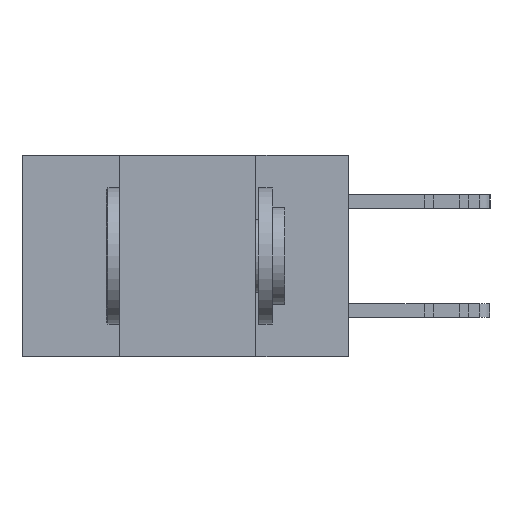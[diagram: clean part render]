
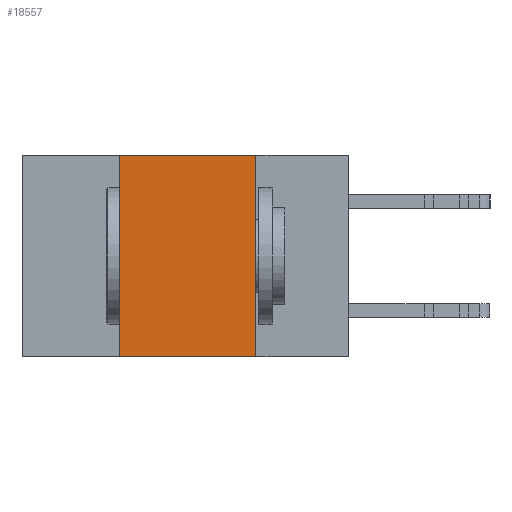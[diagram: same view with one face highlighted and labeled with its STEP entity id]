
A CAD part, left-side view. The second image highlights one B-rep face of the part: STEP entity #18557.
In plain terms, the highlighted planar face has unit normal (-1, 0, 0).
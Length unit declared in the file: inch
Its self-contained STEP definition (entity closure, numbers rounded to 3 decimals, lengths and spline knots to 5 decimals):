
#226 = LINE ( 'NONE', #10860, #3013 ) ;
#1134 = VERTEX_POINT ( 'NONE', #13275 ) ;
#3013 = VECTOR ( 'NONE', #19260, 39.37008 ) ;
#3065 = PLANE ( 'NONE',  #15069 ) ;
#3851 = EDGE_CURVE ( 'NONE', #1134, #13540, #17371, .T. ) ;
#4507 = VECTOR ( 'NONE', #18139, 39.37008 ) ;
#5438 = LINE ( 'NONE', #26823, #4507 ) ;
#6493 = ORIENTED_EDGE ( 'NONE', *, *, #16895, .F. ) ;
#6726 = ORIENTED_EDGE ( 'NONE', *, *, #10129, .F. ) ;
#6945 = DIRECTION ( 'NONE',  ( 1., 0., 0. ) ) ;
#7087 = DIRECTION ( 'NONE',  ( 0., 0., -1. ) ) ;
#8950 = VERTEX_POINT ( 'NONE', #26075 ) ;
#10129 = EDGE_CURVE ( 'NONE', #21380, #13540, #226, .T. ) ;
#10860 = CARTESIAN_POINT ( 'NONE',  ( 0., 0.17, -0.37 ) ) ;
#11260 = CARTESIAN_POINT ( 'NONE',  ( 0., 0.17, 0. ) ) ;
#11976 = ORIENTED_EDGE ( 'NONE', *, *, #14223, .F. ) ;
#12241 = ORIENTED_EDGE ( 'NONE', *, *, #3851, .T. ) ;
#12356 = VECTOR ( 'NONE', #23181, 39.37008 ) ;
#13275 = CARTESIAN_POINT ( 'NONE',  ( 0., 0.42, -0.37 ) ) ;
#13380 = CARTESIAN_POINT ( 'NONE',  ( 0., 0.6, -0.37 ) ) ;
#13540 = VERTEX_POINT ( 'NONE', #27226 ) ;
#14223 = EDGE_CURVE ( 'NONE', #8950, #21380, #21539, .T. ) ;
#15069 = AXIS2_PLACEMENT_3D ( 'NONE', #25850, #6945, #7087 ) ;
#16895 = EDGE_CURVE ( 'NONE', #1134, #8950, #5438, .T. ) ;
#17122 = CARTESIAN_POINT ( 'NONE',  ( 0., 0.6, 0. ) ) ;
#17371 = LINE ( 'NONE', #13380, #23791 ) ;
#18139 = DIRECTION ( 'NONE',  ( 0., 0., 1. ) ) ;
#18557 = ADVANCED_FACE ( 'NONE', ( #25994 ), #3065, .F. ) ;
#19260 = DIRECTION ( 'NONE',  ( 0., 0., -1. ) ) ;
#21380 = VERTEX_POINT ( 'NONE', #11260 ) ;
#21509 = DIRECTION ( 'NONE',  ( 0., -1., 0. ) ) ;
#21539 = LINE ( 'NONE', #17122, #12356 ) ;
#23181 = DIRECTION ( 'NONE',  ( 0., -1., 0. ) ) ;
#23791 = VECTOR ( 'NONE', #21509, 39.37008 ) ;
#24765 = EDGE_LOOP ( 'NONE', ( #6726, #11976, #6493, #12241 ) ) ;
#25850 = CARTESIAN_POINT ( 'NONE',  ( 0., 0.6, 0. ) ) ;
#25994 = FACE_OUTER_BOUND ( 'NONE', #24765, .T. ) ;
#26075 = CARTESIAN_POINT ( 'NONE',  ( 0., 0.42, 0. ) ) ;
#26823 = CARTESIAN_POINT ( 'NONE',  ( 0., 0.42, -0.37 ) ) ;
#27226 = CARTESIAN_POINT ( 'NONE',  ( 0., 0.17, -0.37 ) ) ;
